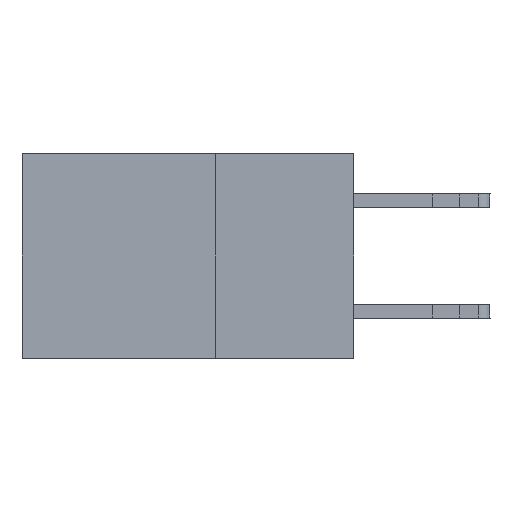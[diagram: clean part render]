
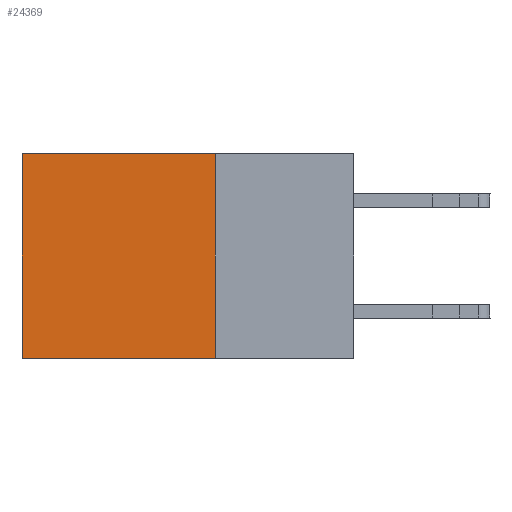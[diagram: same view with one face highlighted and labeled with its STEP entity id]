
A CAD part, left-side view. The second image highlights one B-rep face of the part: STEP entity #24369.
In plain terms, the highlighted planar face has unit normal (-1, 0, 0).
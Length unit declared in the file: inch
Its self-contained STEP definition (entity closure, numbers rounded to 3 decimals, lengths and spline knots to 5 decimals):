
#296 = EDGE_CURVE ( 'NONE', #13730, #5023, #9831, .T. ) ;
#1078 = CARTESIAN_POINT ( 'NONE',  ( 0.2875, 0.25, 0. ) ) ;
#1525 = CARTESIAN_POINT ( 'NONE',  ( 0.2875, 0.6, 0. ) ) ;
#3128 = PLANE ( 'NONE',  #8645 ) ;
#3173 = DIRECTION ( 'NONE',  ( 0., 1., 0. ) ) ;
#4305 = LINE ( 'NONE', #6398, #17850 ) ;
#5023 = VERTEX_POINT ( 'NONE', #24122 ) ;
#6398 = CARTESIAN_POINT ( 'NONE',  ( 0.2875, 0.25, -0.37 ) ) ;
#7322 = EDGE_LOOP ( 'NONE', ( #7797, #21147, #14313, #26032 ) ) ;
#7575 = CARTESIAN_POINT ( 'NONE',  ( 0.2875, 0.25, -0.37 ) ) ;
#7797 = ORIENTED_EDGE ( 'NONE', *, *, #296, .T. ) ;
#8476 = VECTOR ( 'NONE', #3173, 39.37008 ) ;
#8645 = AXIS2_PLACEMENT_3D ( 'NONE', #20360, #20081, #11588 ) ;
#9281 = LINE ( 'NONE', #1078, #8476 ) ;
#9831 = LINE ( 'NONE', #16234, #18515 ) ;
#11588 = DIRECTION ( 'NONE',  ( 0., 0., -1. ) ) ;
#11953 = VECTOR ( 'NONE', #23192, 39.37008 ) ;
#13060 = DIRECTION ( 'NONE',  ( 0., 1., 0. ) ) ;
#13730 = VERTEX_POINT ( 'NONE', #1525 ) ;
#13767 = VERTEX_POINT ( 'NONE', #14029 ) ;
#14029 = CARTESIAN_POINT ( 'NONE',  ( 0.2875, 0.25, 0. ) ) ;
#14145 = DIRECTION ( 'NONE',  ( 0., 0., -1. ) ) ;
#14313 = ORIENTED_EDGE ( 'NONE', *, *, #16369, .F. ) ;
#16234 = CARTESIAN_POINT ( 'NONE',  ( 0.2875, 0.6, 0. ) ) ;
#16369 = EDGE_CURVE ( 'NONE', #13767, #24421, #19033, .T. ) ;
#17850 = VECTOR ( 'NONE', #13060, 39.37008 ) ;
#17982 = EDGE_CURVE ( 'NONE', #13767, #13730, #9281, .T. ) ;
#18515 = VECTOR ( 'NONE', #14145, 39.37008 ) ;
#19033 = LINE ( 'NONE', #23060, #11953 ) ;
#19656 = EDGE_CURVE ( 'NONE', #24421, #5023, #4305, .T. ) ;
#20081 = DIRECTION ( 'NONE',  ( 1., 0., 0. ) ) ;
#20360 = CARTESIAN_POINT ( 'NONE',  ( 0.2875, 0.25, 0. ) ) ;
#21147 = ORIENTED_EDGE ( 'NONE', *, *, #19656, .F. ) ;
#23060 = CARTESIAN_POINT ( 'NONE',  ( 0.2875, 0.25, 0. ) ) ;
#23192 = DIRECTION ( 'NONE',  ( 0., 0., -1. ) ) ;
#24122 = CARTESIAN_POINT ( 'NONE',  ( 0.2875, 0.6, -0.37 ) ) ;
#24369 = ADVANCED_FACE ( 'NONE', ( #24660 ), #3128, .F. ) ;
#24421 = VERTEX_POINT ( 'NONE', #7575 ) ;
#24660 = FACE_OUTER_BOUND ( 'NONE', #7322, .T. ) ;
#26032 = ORIENTED_EDGE ( 'NONE', *, *, #17982, .T. ) ;
